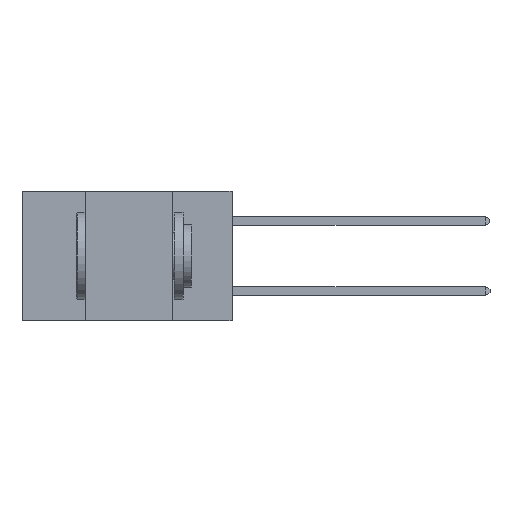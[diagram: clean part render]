
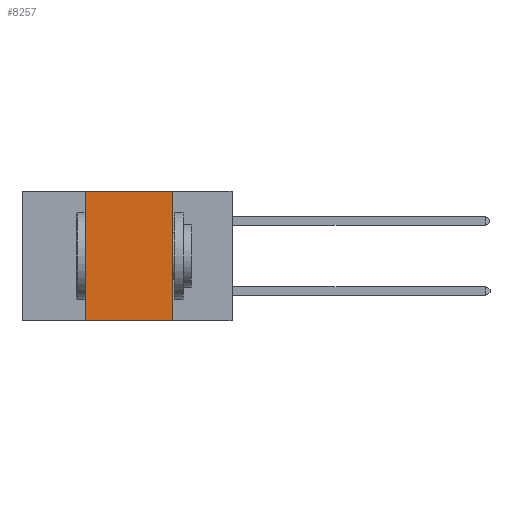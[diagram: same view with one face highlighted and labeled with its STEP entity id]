
A CAD part, left-side view. The second image highlights one B-rep face of the part: STEP entity #8257.
In plain terms, the highlighted planar face has unit normal (-1, 0, 0).
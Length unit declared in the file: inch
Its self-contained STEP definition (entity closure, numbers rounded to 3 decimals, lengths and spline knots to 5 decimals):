
#2469 = EDGE_CURVE ( 'NONE', #3922, #3578, #6991, .T. ) ;
#2631 = EDGE_CURVE ( 'NONE', #3578, #8004, #13406, .T. ) ;
#3310 = VERTEX_POINT ( 'NONE', #22170 ) ;
#3578 = VERTEX_POINT ( 'NONE', #15184 ) ;
#3922 = VERTEX_POINT ( 'NONE', #9933 ) ;
#4239 = VECTOR ( 'NONE', #6677, 39.37008 ) ;
#4599 = CARTESIAN_POINT ( 'NONE',  ( 0., 0.6, 0. ) ) ;
#4686 = ORIENTED_EDGE ( 'NONE', *, *, #5246, .T. ) ;
#5246 = EDGE_CURVE ( 'NONE', #3310, #8004, #6360, .T. ) ;
#5793 = VECTOR ( 'NONE', #11810, 39.37008 ) ;
#6360 = LINE ( 'NONE', #11882, #5793 ) ;
#6403 = CARTESIAN_POINT ( 'NONE',  ( 0., 0.17, 0. ) ) ;
#6465 = VECTOR ( 'NONE', #8225, 39.37008 ) ;
#6474 = CARTESIAN_POINT ( 'NONE',  ( 0., 0.42, 0. ) ) ;
#6677 = DIRECTION ( 'NONE',  ( 0., 0., -1. ) ) ;
#6991 = LINE ( 'NONE', #8259, #6465 ) ;
#7056 = EDGE_LOOP ( 'NONE', ( #13028, #19152, #22290, #4686 ) ) ;
#8004 = VERTEX_POINT ( 'NONE', #15927 ) ;
#8225 = DIRECTION ( 'NONE',  ( 0., -1., 0. ) ) ;
#8257 = ADVANCED_FACE ( 'NONE', ( #16698 ), #16552, .F. ) ;
#8259 = CARTESIAN_POINT ( 'NONE',  ( 0., 0.6, 0. ) ) ;
#9805 = DIRECTION ( 'NONE',  ( 1., 0., 0. ) ) ;
#9933 = CARTESIAN_POINT ( 'NONE',  ( 0., 0.42, 0. ) ) ;
#11810 = DIRECTION ( 'NONE',  ( 0., -1., 0. ) ) ;
#11882 = CARTESIAN_POINT ( 'NONE',  ( 0., 0.6, -0.37 ) ) ;
#13028 = ORIENTED_EDGE ( 'NONE', *, *, #2631, .F. ) ;
#13406 = LINE ( 'NONE', #6403, #4239 ) ;
#15184 = CARTESIAN_POINT ( 'NONE',  ( 0., 0.17, 0. ) ) ;
#15686 = LINE ( 'NONE', #6474, #21865 ) ;
#15691 = AXIS2_PLACEMENT_3D ( 'NONE', #4599, #9805, #21712 ) ;
#15927 = CARTESIAN_POINT ( 'NONE',  ( 0., 0.17, -0.37 ) ) ;
#16552 = PLANE ( 'NONE',  #15691 ) ;
#16581 = DIRECTION ( 'NONE',  ( 0., 0., 1. ) ) ;
#16698 = FACE_OUTER_BOUND ( 'NONE', #7056, .T. ) ;
#17223 = EDGE_CURVE ( 'NONE', #3310, #3922, #15686, .T. ) ;
#19152 = ORIENTED_EDGE ( 'NONE', *, *, #2469, .F. ) ;
#21712 = DIRECTION ( 'NONE',  ( 0., 0., -1. ) ) ;
#21865 = VECTOR ( 'NONE', #16581, 39.37008 ) ;
#22170 = CARTESIAN_POINT ( 'NONE',  ( 0., 0.42, -0.37 ) ) ;
#22290 = ORIENTED_EDGE ( 'NONE', *, *, #17223, .F. ) ;
